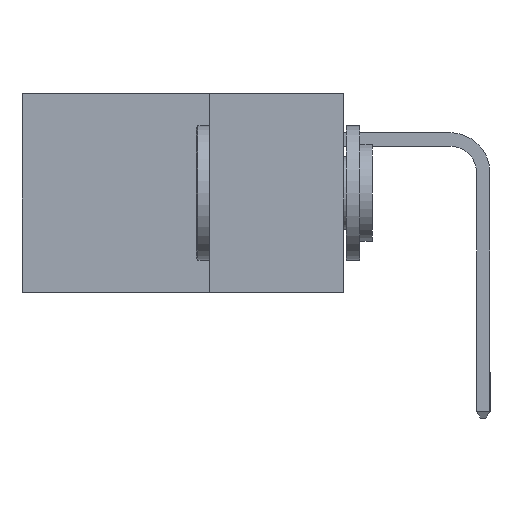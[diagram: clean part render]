
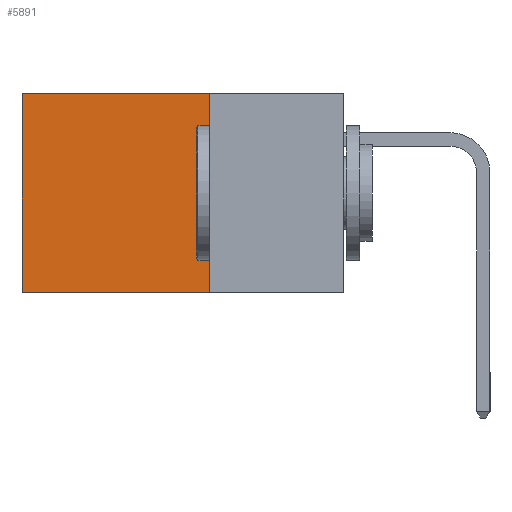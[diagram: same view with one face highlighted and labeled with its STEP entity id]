
A CAD part, left-side view. The second image highlights one B-rep face of the part: STEP entity #5891.
In plain terms, the highlighted planar face has unit normal (-1, 0, 0).
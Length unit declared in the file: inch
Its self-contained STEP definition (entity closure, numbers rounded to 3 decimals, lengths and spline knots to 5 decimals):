
#100 = VERTEX_POINT ( 'NONE', #11373 ) ;
#169 = DIRECTION ( 'NONE',  ( 0., 0., -1. ) ) ;
#468 = CARTESIAN_POINT ( 'NONE',  ( 0.2615, 0.25, -0.37 ) ) ;
#940 = EDGE_CURVE ( 'NONE', #100, #10602, #12369, .T. ) ;
#1154 = CARTESIAN_POINT ( 'NONE',  ( 0.2615, 0.6, -0.37 ) ) ;
#1333 = EDGE_CURVE ( 'NONE', #2456, #8686, #1746, .T. ) ;
#1640 = ORIENTED_EDGE ( 'NONE', *, *, #940, .T. ) ;
#1746 = LINE ( 'NONE', #12567, #6249 ) ;
#2456 = VERTEX_POINT ( 'NONE', #13087 ) ;
#2535 = VECTOR ( 'NONE', #13074, 39.37008 ) ;
#2672 = LINE ( 'NONE', #10042, #2535 ) ;
#2748 = CARTESIAN_POINT ( 'NONE',  ( 0.2615, 0.25, 0. ) ) ;
#3327 = FACE_OUTER_BOUND ( 'NONE', #5902, .T. ) ;
#3567 = LINE ( 'NONE', #468, #13112 ) ;
#4209 = VECTOR ( 'NONE', #11322, 39.37008 ) ;
#4695 = AXIS2_PLACEMENT_3D ( 'NONE', #9728, #9801, #169 ) ;
#5439 = PLANE ( 'NONE',  #4695 ) ;
#5891 = ADVANCED_FACE ( 'NONE', ( #3327 ), #5439, .F. ) ;
#5902 = EDGE_LOOP ( 'NONE', ( #11257, #10826, #12052, #1640 ) ) ;
#5940 = DIRECTION ( 'NONE',  ( 0., 0., -1. ) ) ;
#6158 = DIRECTION ( 'NONE',  ( 0., 1., 0. ) ) ;
#6249 = VECTOR ( 'NONE', #6158, 39.37008 ) ;
#8686 = VERTEX_POINT ( 'NONE', #1154 ) ;
#9173 = EDGE_CURVE ( 'NONE', #10602, #8686, #2672, .T. ) ;
#9728 = CARTESIAN_POINT ( 'NONE',  ( 0.2615, 0.25, -0.37 ) ) ;
#9801 = DIRECTION ( 'NONE',  ( 1., 0., 0. ) ) ;
#10042 = CARTESIAN_POINT ( 'NONE',  ( 0.2615, 0.6, -0.37 ) ) ;
#10113 = CARTESIAN_POINT ( 'NONE',  ( 0.2615, 0.6, 0. ) ) ;
#10602 = VERTEX_POINT ( 'NONE', #10113 ) ;
#10826 = ORIENTED_EDGE ( 'NONE', *, *, #1333, .F. ) ;
#11257 = ORIENTED_EDGE ( 'NONE', *, *, #9173, .T. ) ;
#11322 = DIRECTION ( 'NONE',  ( 0., 1., 0. ) ) ;
#11373 = CARTESIAN_POINT ( 'NONE',  ( 0.2615, 0.25, 0. ) ) ;
#12052 = ORIENTED_EDGE ( 'NONE', *, *, #12458, .F. ) ;
#12369 = LINE ( 'NONE', #2748, #4209 ) ;
#12458 = EDGE_CURVE ( 'NONE', #100, #2456, #3567, .T. ) ;
#12567 = CARTESIAN_POINT ( 'NONE',  ( 0.2615, 0.25, -0.37 ) ) ;
#13074 = DIRECTION ( 'NONE',  ( 0., 0., -1. ) ) ;
#13087 = CARTESIAN_POINT ( 'NONE',  ( 0.2615, 0.25, -0.37 ) ) ;
#13112 = VECTOR ( 'NONE', #5940, 39.37008 ) ;
